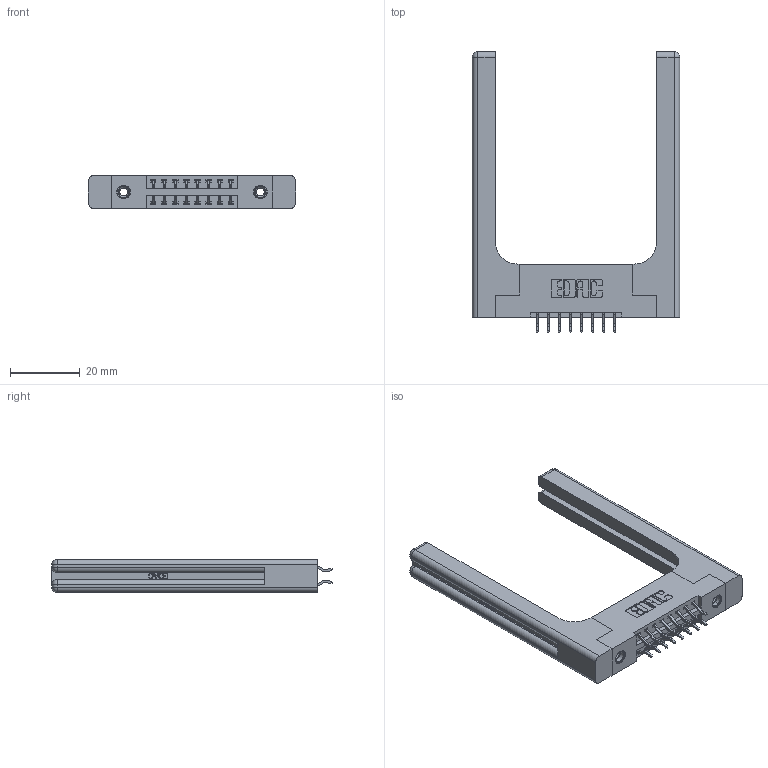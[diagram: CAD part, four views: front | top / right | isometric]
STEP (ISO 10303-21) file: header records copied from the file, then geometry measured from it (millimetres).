
FILE_DESCRIPTION (( 'STEP AP203' ), '1' );
FILE_NAME ('396-016-556-258.STEP', '2019-10-30T02:41:23', ( '' ), ( '' ), 'SwSTEP 2.0', 'SolidWorks 2016', '' );
FILE_SCHEMA (( 'CONFIG_CONTROL_DESIGN' ));
Length unit declared in the file: inch
Products named in the file (5): 346 Part_Flush Mounting Lugs - 0.156 Dia-TH; 346-220-058_345-220-058; 345-292-001_556 Tail; 345-250-001_345-250-001-102; 396-016-556-258
Assembly tree (21 placements, depth 2):
  396-016-556-258
    346 Part_Flush Mounting Lugs - 0.156 Dia-TH
    345-292-001_556 Tail  x16
    345-250-001_345-250-001-102  x2
    346-220-058_345-220-058  x2
Bounding box: 59.46 x 80.53 x 9.4 mm (x, y, z)
Volume: 13027.8 mm3; surface area: 12029.7 mm2
Topology: 21 solids, 21 shells, 1306 faces, 3763 edges, 2466 vertices
Faces by surface type: plane 848, cylinder 398, bspline 36, cone 12, sphere 8, torus 4
Entity records: 15200 total; most frequent: CARTESIAN_POINT 3573, ORIENTED_EDGE 2292, DIRECTION 2122, EDGE_CURVE 1146, LINE 882, VECTOR 882, VERTEX_POINT 754, AXIS2_PLACEMENT_3D 620
